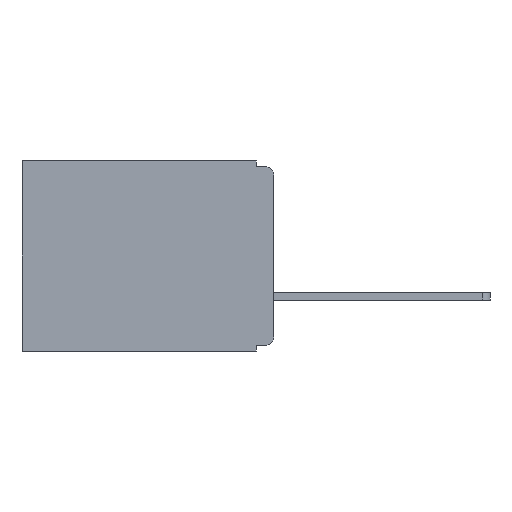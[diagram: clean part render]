
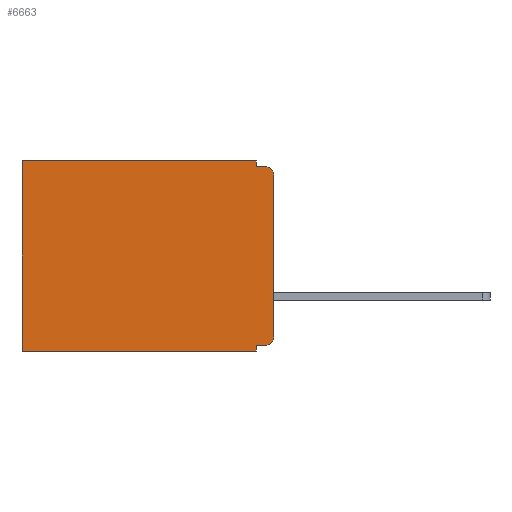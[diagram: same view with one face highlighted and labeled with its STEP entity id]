
A CAD part, left-side view. The second image highlights one B-rep face of the part: STEP entity #6663.
In plain terms, the highlighted planar face has unit normal (-1, 0, 0).
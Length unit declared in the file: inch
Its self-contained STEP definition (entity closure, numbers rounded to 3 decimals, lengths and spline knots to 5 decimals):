
#49 = VERTEX_POINT ( 'NONE', #1998 ) ;
#130 = VECTOR ( 'NONE', #10705, 39.37008 ) ;
#217 = DIRECTION ( 'NONE',  ( 0., 0., -1. ) ) ;
#350 = AXIS2_PLACEMENT_3D ( 'NONE', #6555, #6226, #1193 ) ;
#438 = CARTESIAN_POINT ( 'NONE',  ( 0.3, 0., -0.33 ) ) ;
#694 = LINE ( 'NONE', #835, #8955 ) ;
#812 = VECTOR ( 'NONE', #217, 39.37008 ) ;
#835 = CARTESIAN_POINT ( 'NONE',  ( 0.3, 0.437, -0.33 ) ) ;
#934 = LINE ( 'NONE', #9908, #9156 ) ;
#1131 = LINE ( 'NONE', #6084, #6521 ) ;
#1193 = DIRECTION ( 'NONE',  ( 0., 0., -1. ) ) ;
#1450 = VECTOR ( 'NONE', #11922, 39.37008 ) ;
#1796 = VERTEX_POINT ( 'NONE', #5509 ) ;
#1930 = CARTESIAN_POINT ( 'NONE',  ( 0.3, 0.031, 0. ) ) ;
#1998 = CARTESIAN_POINT ( 'NONE',  ( 0.3, 0.031, -0.33 ) ) ;
#2334 = ORIENTED_EDGE ( 'NONE', *, *, #4187, .T. ) ;
#2724 = DIRECTION ( 'NONE',  ( 0., 1., 0. ) ) ;
#2808 = VERTEX_POINT ( 'NONE', #9984 ) ;
#3055 = CARTESIAN_POINT ( 'NONE',  ( 0.3, 0.015, -0.305 ) ) ;
#3060 = ORIENTED_EDGE ( 'NONE', *, *, #5693, .F. ) ;
#3069 = CARTESIAN_POINT ( 'NONE',  ( 0.3, 0.437, -0.33 ) ) ;
#3394 = VERTEX_POINT ( 'NONE', #10211 ) ;
#3833 = EDGE_CURVE ( 'NONE', #6562, #3394, #1131, .T. ) ;
#3947 = EDGE_CURVE ( 'NONE', #6477, #1796, #12063, .T. ) ;
#4130 = EDGE_CURVE ( 'NONE', #8286, #4371, #9562, .T. ) ;
#4187 = EDGE_CURVE ( 'NONE', #6562, #1796, #9034, .T. ) ;
#4287 = EDGE_CURVE ( 'NONE', #8286, #3394, #9929, .T. ) ;
#4371 = VERTEX_POINT ( 'NONE', #12017 ) ;
#4971 = DIRECTION ( 'NONE',  ( 0., 0., -1. ) ) ;
#5509 = CARTESIAN_POINT ( 'NONE',  ( 0.3, 0.015, -0.01 ) ) ;
#5514 = EDGE_CURVE ( 'NONE', #49, #7429, #9202, .T. ) ;
#5579 = ORIENTED_EDGE ( 'NONE', *, *, #3947, .F. ) ;
#5618 = EDGE_LOOP ( 'NONE', ( #6613, #2334, #5579, #3060, #8329, #6343, #6179, #11791, #11702, #6846 ) ) ;
#5693 = EDGE_CURVE ( 'NONE', #11335, #6477, #9325, .T. ) ;
#5753 = EDGE_CURVE ( 'NONE', #4371, #49, #6166, .T. ) ;
#5809 = CARTESIAN_POINT ( 'NONE',  ( 0.3, 0., -0.025 ) ) ;
#5853 = CARTESIAN_POINT ( 'NONE',  ( 0.3, 0.031, -0.01 ) ) ;
#6006 = VECTOR ( 'NONE', #2724, 39.37008 ) ;
#6084 = CARTESIAN_POINT ( 'NONE',  ( 0.3, 0., -0.33 ) ) ;
#6166 = LINE ( 'NONE', #10291, #130 ) ;
#6179 = ORIENTED_EDGE ( 'NONE', *, *, #5514, .F. ) ;
#6226 = DIRECTION ( 'NONE',  ( 1., 0., 0. ) ) ;
#6343 = ORIENTED_EDGE ( 'NONE', *, *, #9721, .T. ) ;
#6477 = VERTEX_POINT ( 'NONE', #5853 ) ;
#6521 = VECTOR ( 'NONE', #4971, 39.37008 ) ;
#6555 = CARTESIAN_POINT ( 'NONE',  ( 0.3, 0., -0.33 ) ) ;
#6562 = VERTEX_POINT ( 'NONE', #5809 ) ;
#6613 = ORIENTED_EDGE ( 'NONE', *, *, #3833, .F. ) ;
#6663 = ADVANCED_FACE ( 'NONE', ( #11933 ), #11604, .F. ) ;
#6846 = ORIENTED_EDGE ( 'NONE', *, *, #4287, .T. ) ;
#6856 = EDGE_CURVE ( 'NONE', #11335, #2808, #934, .T. ) ;
#7384 = CARTESIAN_POINT ( 'NONE',  ( 0.3, 0., -0.01 ) ) ;
#7420 = VECTOR ( 'NONE', #11655, 39.37008 ) ;
#7429 = VERTEX_POINT ( 'NONE', #3069 ) ;
#8286 = VERTEX_POINT ( 'NONE', #8936 ) ;
#8329 = ORIENTED_EDGE ( 'NONE', *, *, #6856, .T. ) ;
#8661 = AXIS2_PLACEMENT_3D ( 'NONE', #3055, #11760, #11720 ) ;
#8936 = CARTESIAN_POINT ( 'NONE',  ( 0.3, 0.015, -0.32 ) ) ;
#8955 = VECTOR ( 'NONE', #10970, 39.37008 ) ;
#9019 = AXIS2_PLACEMENT_3D ( 'NONE', #10971, #11078, #11115 ) ;
#9034 = CIRCLE ( 'NONE', #9019, 0.015 ) ;
#9156 = VECTOR ( 'NONE', #9969, 39.37008 ) ;
#9202 = LINE ( 'NONE', #438, #6006 ) ;
#9325 = LINE ( 'NONE', #11737, #812 ) ;
#9562 = LINE ( 'NONE', #9994, #1450 ) ;
#9721 = EDGE_CURVE ( 'NONE', #2808, #7429, #694, .T. ) ;
#9908 = CARTESIAN_POINT ( 'NONE',  ( 0.3, 0., 0. ) ) ;
#9929 = CIRCLE ( 'NONE', #8661, 0.015 ) ;
#9969 = DIRECTION ( 'NONE',  ( 0., 1., 0. ) ) ;
#9984 = CARTESIAN_POINT ( 'NONE',  ( 0.3, 0.437, 0. ) ) ;
#9994 = CARTESIAN_POINT ( 'NONE',  ( 0.3, 0., -0.32 ) ) ;
#10211 = CARTESIAN_POINT ( 'NONE',  ( 0.3, 0., -0.305 ) ) ;
#10291 = CARTESIAN_POINT ( 'NONE',  ( 0.3, 0.031, -0.33 ) ) ;
#10705 = DIRECTION ( 'NONE',  ( 0., 0., -1. ) ) ;
#10970 = DIRECTION ( 'NONE',  ( 0., 0., -1. ) ) ;
#10971 = CARTESIAN_POINT ( 'NONE',  ( 0.3, 0.015, -0.025 ) ) ;
#11078 = DIRECTION ( 'NONE',  ( -1., 0., 0. ) ) ;
#11115 = DIRECTION ( 'NONE',  ( 0., 0., -1. ) ) ;
#11335 = VERTEX_POINT ( 'NONE', #1930 ) ;
#11604 = PLANE ( 'NONE',  #350 ) ;
#11655 = DIRECTION ( 'NONE',  ( 0., -1., 0. ) ) ;
#11702 = ORIENTED_EDGE ( 'NONE', *, *, #4130, .F. ) ;
#11720 = DIRECTION ( 'NONE',  ( 0., 0., -1. ) ) ;
#11737 = CARTESIAN_POINT ( 'NONE',  ( 0.3, 0.031, 0. ) ) ;
#11760 = DIRECTION ( 'NONE',  ( -1., 0., 0. ) ) ;
#11791 = ORIENTED_EDGE ( 'NONE', *, *, #5753, .F. ) ;
#11922 = DIRECTION ( 'NONE',  ( 0., 1., 0. ) ) ;
#11933 = FACE_OUTER_BOUND ( 'NONE', #5618, .T. ) ;
#12017 = CARTESIAN_POINT ( 'NONE',  ( 0.3, 0.031, -0.32 ) ) ;
#12063 = LINE ( 'NONE', #7384, #7420 ) ;
